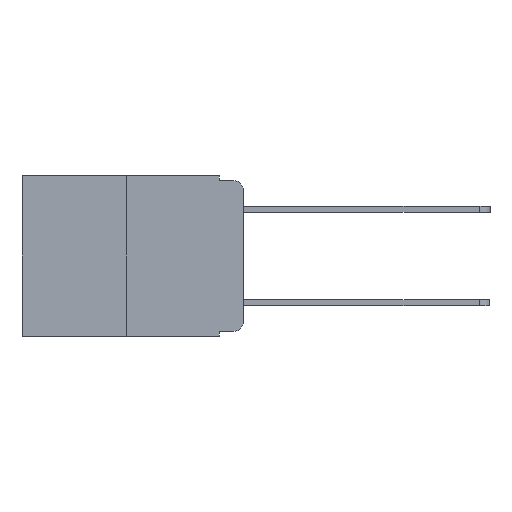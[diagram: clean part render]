
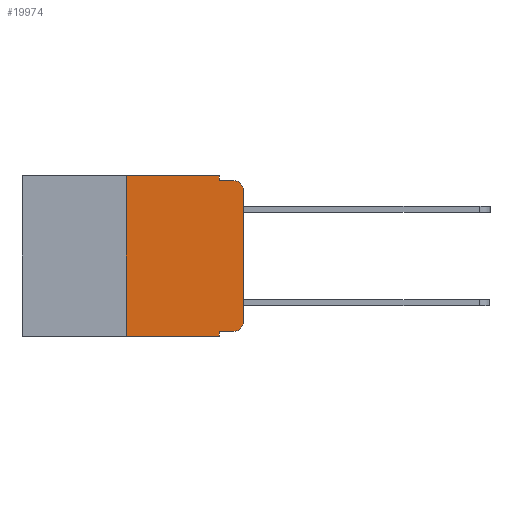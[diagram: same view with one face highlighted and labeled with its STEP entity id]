
A CAD part, left-side view. The second image highlights one B-rep face of the part: STEP entity #19974.
In plain terms, the highlighted planar face has unit normal (-1, 0, 0).
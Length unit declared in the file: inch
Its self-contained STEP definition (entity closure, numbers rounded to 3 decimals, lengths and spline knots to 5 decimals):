
#26 = CARTESIAN_POINT ( 'NONE',  ( 0., 0.02, -0.01 ) ) ;
#80 = LINE ( 'NONE', #1778, #4568 ) ;
#155 = DIRECTION ( 'NONE',  ( -1., 0., 0. ) ) ;
#186 = VERTEX_POINT ( 'NONE', #26 ) ;
#798 = CARTESIAN_POINT ( 'NONE',  ( 0., 0.051, -0.01 ) ) ;
#1006 = DIRECTION ( 'NONE',  ( 0., -1., 0. ) ) ;
#1084 = LINE ( 'NONE', #21308, #18782 ) ;
#1582 = EDGE_LOOP ( 'NONE', ( #21662, #7459, #6003, #12514, #19072, #18266, #4396, #4030, #8989, #3735 ) ) ;
#1778 = CARTESIAN_POINT ( 'NONE',  ( 0., 0.473, -0.343 ) ) ;
#2269 = EDGE_CURVE ( 'NONE', #20345, #23094, #13823, .T. ) ;
#2601 = EDGE_CURVE ( 'NONE', #11039, #22787, #7021, .T. ) ;
#2717 = VECTOR ( 'NONE', #12260, 39.37008 ) ;
#3076 = EDGE_CURVE ( 'NONE', #20345, #21964, #80, .T. ) ;
#3494 = VECTOR ( 'NONE', #14369, 39.37008 ) ;
#3681 = DIRECTION ( 'NONE',  ( 0., -1., 0. ) ) ;
#3735 = ORIENTED_EDGE ( 'NONE', *, *, #22808, .T. ) ;
#3960 = VERTEX_POINT ( 'NONE', #17506 ) ;
#4030 = ORIENTED_EDGE ( 'NONE', *, *, #5301, .F. ) ;
#4290 = DIRECTION ( 'NONE',  ( 0., 0., -1. ) ) ;
#4357 = VERTEX_POINT ( 'NONE', #22146 ) ;
#4396 = ORIENTED_EDGE ( 'NONE', *, *, #3076, .T. ) ;
#4541 = AXIS2_PLACEMENT_3D ( 'NONE', #11341, #155, #13152 ) ;
#4568 = VECTOR ( 'NONE', #3681, 39.37008 ) ;
#4603 = CARTESIAN_POINT ( 'NONE',  ( 0., 0.473, 0. ) ) ;
#4713 = DIRECTION ( 'NONE',  ( -1., 0., 0. ) ) ;
#4993 = LINE ( 'NONE', #10302, #18305 ) ;
#5209 = CARTESIAN_POINT ( 'NONE',  ( 0., 0.25, 0. ) ) ;
#5301 = EDGE_CURVE ( 'NONE', #4357, #21964, #10004, .T. ) ;
#5501 = VERTEX_POINT ( 'NONE', #12806 ) ;
#6003 = ORIENTED_EDGE ( 'NONE', *, *, #22909, .F. ) ;
#6495 = DIRECTION ( 'NONE',  ( 0., 0., -1. ) ) ;
#6849 = DIRECTION ( 'NONE',  ( 0., -1., 0. ) ) ;
#7021 = LINE ( 'NONE', #18767, #20188 ) ;
#7219 = CIRCLE ( 'NONE', #4541, 0.02 ) ;
#7459 = ORIENTED_EDGE ( 'NONE', *, *, #17784, .T. ) ;
#7955 = LINE ( 'NONE', #8651, #21602 ) ;
#8354 = EDGE_CURVE ( 'NONE', #5501, #3960, #1084, .T. ) ;
#8651 = CARTESIAN_POINT ( 'NONE',  ( 0., 0.051, -0.01 ) ) ;
#8989 = ORIENTED_EDGE ( 'NONE', *, *, #20673, .T. ) ;
#9493 = LINE ( 'NONE', #22879, #18966 ) ;
#10004 = LINE ( 'NONE', #19359, #2717 ) ;
#10048 = VERTEX_POINT ( 'NONE', #12109 ) ;
#10096 = PLANE ( 'NONE',  #11951 ) ;
#10202 = CARTESIAN_POINT ( 'NONE',  ( 0., 0.051, 0. ) ) ;
#10302 = CARTESIAN_POINT ( 'NONE',  ( 0., 0.051, -0.333 ) ) ;
#10894 = CARTESIAN_POINT ( 'NONE',  ( 0., 0.25, 0. ) ) ;
#11039 = VERTEX_POINT ( 'NONE', #10202 ) ;
#11341 = CARTESIAN_POINT ( 'NONE',  ( 0., 0.02, -0.03 ) ) ;
#11951 = AXIS2_PLACEMENT_3D ( 'NONE', #4603, #17319, #6495 ) ;
#12109 = CARTESIAN_POINT ( 'NONE',  ( 0., 0.02, -0.333 ) ) ;
#12260 = DIRECTION ( 'NONE',  ( 0., 0., -1. ) ) ;
#12514 = ORIENTED_EDGE ( 'NONE', *, *, #2601, .F. ) ;
#12806 = CARTESIAN_POINT ( 'NONE',  ( 0., 0., -0.313 ) ) ;
#12911 = CARTESIAN_POINT ( 'NONE',  ( 0., 0.051, -0.343 ) ) ;
#13152 = DIRECTION ( 'NONE',  ( 0., 0., -1. ) ) ;
#13823 = LINE ( 'NONE', #5209, #3494 ) ;
#14369 = DIRECTION ( 'NONE',  ( 0., 0., 1. ) ) ;
#15634 = CARTESIAN_POINT ( 'NONE',  ( 0., 0.02, -0.313 ) ) ;
#16145 = FACE_OUTER_BOUND ( 'NONE', #1582, .T. ) ;
#17319 = DIRECTION ( 'NONE',  ( 1., 0., 0. ) ) ;
#17425 = DIRECTION ( 'NONE',  ( 0., 0., -1. ) ) ;
#17506 = CARTESIAN_POINT ( 'NONE',  ( 0., 0., -0.03 ) ) ;
#17557 = AXIS2_PLACEMENT_3D ( 'NONE', #15634, #4713, #17425 ) ;
#17609 = DIRECTION ( 'NONE',  ( 0., -1., 0. ) ) ;
#17784 = EDGE_CURVE ( 'NONE', #3960, #186, #7219, .T. ) ;
#18108 = EDGE_CURVE ( 'NONE', #23094, #11039, #9493, .T. ) ;
#18266 = ORIENTED_EDGE ( 'NONE', *, *, #2269, .F. ) ;
#18305 = VECTOR ( 'NONE', #1006, 39.37008 ) ;
#18767 = CARTESIAN_POINT ( 'NONE',  ( 0., 0.051, 0. ) ) ;
#18782 = VECTOR ( 'NONE', #23047, 39.37008 ) ;
#18966 = VECTOR ( 'NONE', #17609, 39.37008 ) ;
#19072 = ORIENTED_EDGE ( 'NONE', *, *, #18108, .F. ) ;
#19133 = CIRCLE ( 'NONE', #17557, 0.02 ) ;
#19359 = CARTESIAN_POINT ( 'NONE',  ( 0., 0.051, 0. ) ) ;
#19974 = ADVANCED_FACE ( 'NONE', ( #16145 ), #10096, .F. ) ;
#20188 = VECTOR ( 'NONE', #4290, 39.37008 ) ;
#20345 = VERTEX_POINT ( 'NONE', #21894 ) ;
#20673 = EDGE_CURVE ( 'NONE', #4357, #10048, #4993, .T. ) ;
#21308 = CARTESIAN_POINT ( 'NONE',  ( 0., 0., 0. ) ) ;
#21602 = VECTOR ( 'NONE', #6849, 39.37008 ) ;
#21662 = ORIENTED_EDGE ( 'NONE', *, *, #8354, .T. ) ;
#21894 = CARTESIAN_POINT ( 'NONE',  ( 0., 0.25, -0.343 ) ) ;
#21964 = VERTEX_POINT ( 'NONE', #12911 ) ;
#22146 = CARTESIAN_POINT ( 'NONE',  ( 0., 0.051, -0.333 ) ) ;
#22787 = VERTEX_POINT ( 'NONE', #798 ) ;
#22808 = EDGE_CURVE ( 'NONE', #10048, #5501, #19133, .T. ) ;
#22879 = CARTESIAN_POINT ( 'NONE',  ( 0., 0.473, 0. ) ) ;
#22909 = EDGE_CURVE ( 'NONE', #22787, #186, #7955, .T. ) ;
#23047 = DIRECTION ( 'NONE',  ( 0., 0., 1. ) ) ;
#23094 = VERTEX_POINT ( 'NONE', #10894 ) ;
